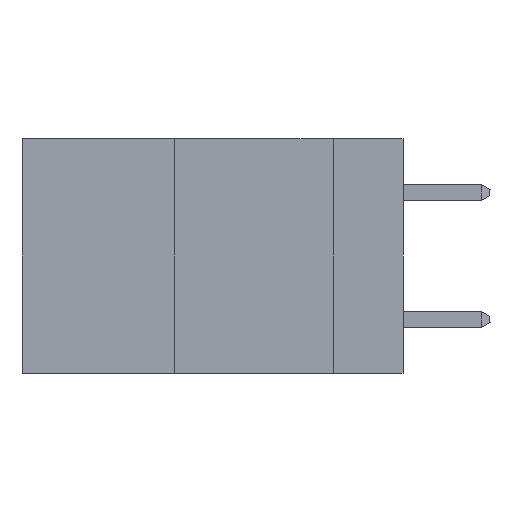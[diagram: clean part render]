
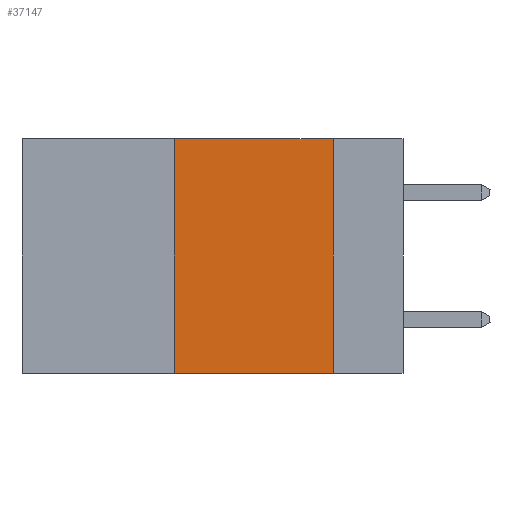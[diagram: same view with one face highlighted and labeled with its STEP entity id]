
A CAD part, left-side view. The second image highlights one B-rep face of the part: STEP entity #37147.
In plain terms, the highlighted planar face has unit normal (-1, 0, 0).
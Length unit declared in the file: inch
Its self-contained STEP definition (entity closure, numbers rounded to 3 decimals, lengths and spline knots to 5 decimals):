
#394 = VECTOR ( 'NONE', #19217, 39.37008 ) ;
#1576 = ORIENTED_EDGE ( 'NONE', *, *, #18046, .F. ) ;
#3005 = CARTESIAN_POINT ( 'NONE',  ( 0., 0.11, 0. ) ) ;
#5390 = CARTESIAN_POINT ( 'NONE',  ( 0., 0.6, 0. ) ) ;
#5765 = CARTESIAN_POINT ( 'NONE',  ( 0., 0.36, 0. ) ) ;
#6283 = CARTESIAN_POINT ( 'NONE',  ( 0., 0.36, -0.37 ) ) ;
#7467 = VERTEX_POINT ( 'NONE', #13186 ) ;
#8034 = EDGE_CURVE ( 'NONE', #7467, #34366, #42083, .T. ) ;
#8580 = EDGE_CURVE ( 'NONE', #34366, #30642, #42557, .T. ) ;
#9636 = VECTOR ( 'NONE', #26968, 39.37008 ) ;
#10013 = CARTESIAN_POINT ( 'NONE',  ( 0., 0.6, 0. ) ) ;
#13186 = CARTESIAN_POINT ( 'NONE',  ( 0., 0.36, 0. ) ) ;
#18046 = EDGE_CURVE ( 'NONE', #33890, #7467, #39931, .T. ) ;
#18575 = ORIENTED_EDGE ( 'NONE', *, *, #8580, .F. ) ;
#19217 = DIRECTION ( 'NONE',  ( 0., 0., -1. ) ) ;
#20204 = CARTESIAN_POINT ( 'NONE',  ( 0., 0.6, -0.37 ) ) ;
#20670 = ORIENTED_EDGE ( 'NONE', *, *, #8034, .F. ) ;
#22626 = FACE_OUTER_BOUND ( 'NONE', #30722, .T. ) ;
#23042 = DIRECTION ( 'NONE',  ( 0., 0., 1. ) ) ;
#24194 = EDGE_CURVE ( 'NONE', #33890, #30642, #42290, .T. ) ;
#25700 = PLANE ( 'NONE',  #40188 ) ;
#26725 = DIRECTION ( 'NONE',  ( 0., -1., 0. ) ) ;
#26968 = DIRECTION ( 'NONE',  ( 0., -1., 0. ) ) ;
#30642 = VERTEX_POINT ( 'NONE', #31962 ) ;
#30722 = EDGE_LOOP ( 'NONE', ( #18575, #20670, #1576, #36390 ) ) ;
#31962 = CARTESIAN_POINT ( 'NONE',  ( 0., 0.11, -0.37 ) ) ;
#33890 = VERTEX_POINT ( 'NONE', #6283 ) ;
#34366 = VERTEX_POINT ( 'NONE', #41821 ) ;
#36390 = ORIENTED_EDGE ( 'NONE', *, *, #24194, .T. ) ;
#37147 = ADVANCED_FACE ( 'NONE', ( #22626 ), #25700, .F. ) ;
#37805 = VECTOR ( 'NONE', #23042, 39.37008 ) ;
#39774 = DIRECTION ( 'NONE',  ( 0., 0., -1. ) ) ;
#39931 = LINE ( 'NONE', #5765, #37805 ) ;
#40188 = AXIS2_PLACEMENT_3D ( 'NONE', #5390, #43025, #39774 ) ;
#41022 = VECTOR ( 'NONE', #26725, 39.37008 ) ;
#41821 = CARTESIAN_POINT ( 'NONE',  ( 0., 0.11, 0. ) ) ;
#42083 = LINE ( 'NONE', #10013, #41022 ) ;
#42290 = LINE ( 'NONE', #20204, #9636 ) ;
#42557 = LINE ( 'NONE', #3005, #394 ) ;
#43025 = DIRECTION ( 'NONE',  ( 1., 0., 0. ) ) ;
